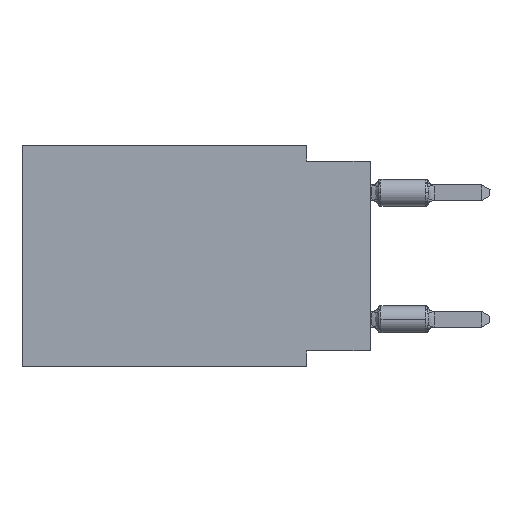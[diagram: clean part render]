
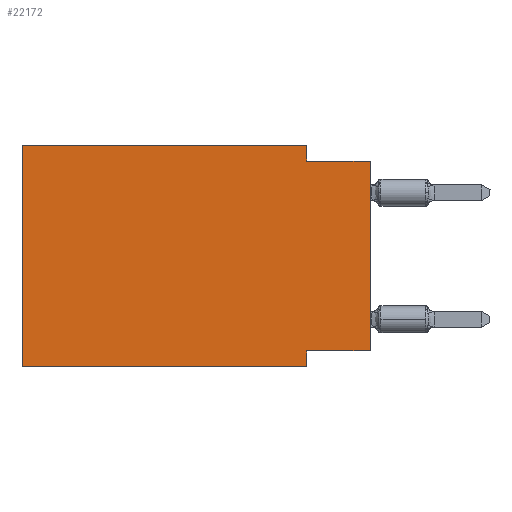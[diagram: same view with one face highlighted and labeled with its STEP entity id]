
A CAD part, left-side view. The second image highlights one B-rep face of the part: STEP entity #22172.
In plain terms, the highlighted planar face has unit normal (-1, 0, 0).
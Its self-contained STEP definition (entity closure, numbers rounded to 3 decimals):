
#338 = VECTOR ( 'NONE', #21664, 1000. ) ;
#399 = VERTEX_POINT ( 'NONE', #14264 ) ;
#623 = LINE ( 'NONE', #23967, #23879 ) ;
#987 = VERTEX_POINT ( 'NONE', #2656 ) ;
#2633 = CARTESIAN_POINT ( 'NONE',  ( 0., 13.97, 0. ) ) ;
#2656 = CARTESIAN_POINT ( 'NONE',  ( 0., 13.97, -8.89 ) ) ;
#2758 = EDGE_CURVE ( 'NONE', #3382, #399, #11212, .T. ) ;
#3339 = FACE_OUTER_BOUND ( 'NONE', #24590, .T. ) ;
#3382 = VERTEX_POINT ( 'NONE', #27331 ) ;
#3760 = VECTOR ( 'NONE', #12024, 1000. ) ;
#4665 = CARTESIAN_POINT ( 'NONE',  ( 0., 0., 0. ) ) ;
#5239 = LINE ( 'NONE', #24772, #11299 ) ;
#5345 = VERTEX_POINT ( 'NONE', #9623 ) ;
#5519 = DIRECTION ( 'NONE',  ( 0., 0., 1. ) ) ;
#6769 = VECTOR ( 'NONE', #18265, 1000. ) ;
#6833 = ORIENTED_EDGE ( 'NONE', *, *, #20634, .F. ) ;
#6986 = DIRECTION ( 'NONE',  ( 0., -1., 0. ) ) ;
#7038 = LINE ( 'NONE', #4665, #338 ) ;
#7321 = CARTESIAN_POINT ( 'NONE',  ( 0., 2.54, 0. ) ) ;
#7793 = ORIENTED_EDGE ( 'NONE', *, *, #2758, .F. ) ;
#8120 = DIRECTION ( 'NONE',  ( 0., 0., -1. ) ) ;
#8438 = ORIENTED_EDGE ( 'NONE', *, *, #23819, .F. ) ;
#8537 = EDGE_CURVE ( 'NONE', #23138, #5345, #18542, .T. ) ;
#9420 = ORIENTED_EDGE ( 'NONE', *, *, #10108, .F. ) ;
#9623 = CARTESIAN_POINT ( 'NONE',  ( 0., 2.54, -8.255 ) ) ;
#9711 = AXIS2_PLACEMENT_3D ( 'NONE', #18797, #27377, #8120 ) ;
#9841 = ORIENTED_EDGE ( 'NONE', *, *, #23227, .T. ) ;
#9898 = VECTOR ( 'NONE', #18195, 1000. ) ;
#10108 = EDGE_CURVE ( 'NONE', #399, #18042, #10135, .T. ) ;
#10135 = LINE ( 'NONE', #7321, #17429 ) ;
#11049 = DIRECTION ( 'NONE',  ( 0., -1., 0. ) ) ;
#11212 = LINE ( 'NONE', #2633, #22185 ) ;
#11299 = VECTOR ( 'NONE', #5519, 1000. ) ;
#11403 = ORIENTED_EDGE ( 'NONE', *, *, #8537, .F. ) ;
#12024 = DIRECTION ( 'NONE',  ( 0., 0., -1. ) ) ;
#12200 = CARTESIAN_POINT ( 'NONE',  ( 0., 0., -0.635 ) ) ;
#12247 = CARTESIAN_POINT ( 'NONE',  ( 0., 2.54, -8.89 ) ) ;
#14264 = CARTESIAN_POINT ( 'NONE',  ( 0., 2.54, 0. ) ) ;
#14389 = LINE ( 'NONE', #20724, #9898 ) ;
#16452 = VERTEX_POINT ( 'NONE', #12247 ) ;
#17429 = VECTOR ( 'NONE', #22637, 1000. ) ;
#17592 = ORIENTED_EDGE ( 'NONE', *, *, #17677, .F. ) ;
#17677 = EDGE_CURVE ( 'NONE', #18042, #27198, #623, .T. ) ;
#18042 = VERTEX_POINT ( 'NONE', #24445 ) ;
#18195 = DIRECTION ( 'NONE',  ( 0., -1., 0. ) ) ;
#18265 = DIRECTION ( 'NONE',  ( 0., 1., 0. ) ) ;
#18542 = LINE ( 'NONE', #26701, #6769 ) ;
#18797 = CARTESIAN_POINT ( 'NONE',  ( 0., 13.97, 0. ) ) ;
#18990 = EDGE_CURVE ( 'NONE', #987, #16452, #14389, .T. ) ;
#19153 = CARTESIAN_POINT ( 'NONE',  ( 0., 0., -8.255 ) ) ;
#19332 = ORIENTED_EDGE ( 'NONE', *, *, #18990, .T. ) ;
#20634 = EDGE_CURVE ( 'NONE', #987, #3382, #5239, .T. ) ;
#20724 = CARTESIAN_POINT ( 'NONE',  ( 0., 13.97, -8.89 ) ) ;
#21019 = CARTESIAN_POINT ( 'NONE',  ( 0., 2.54, -8.89 ) ) ;
#21664 = DIRECTION ( 'NONE',  ( 0., 0., 1. ) ) ;
#22172 = ADVANCED_FACE ( 'NONE', ( #3339 ), #24980, .F. ) ;
#22185 = VECTOR ( 'NONE', #6986, 1000. ) ;
#22637 = DIRECTION ( 'NONE',  ( 0., 0., -1. ) ) ;
#23138 = VERTEX_POINT ( 'NONE', #19153 ) ;
#23227 = EDGE_CURVE ( 'NONE', #23138, #27198, #7038, .T. ) ;
#23819 = EDGE_CURVE ( 'NONE', #5345, #16452, #25094, .T. ) ;
#23879 = VECTOR ( 'NONE', #11049, 1000. ) ;
#23967 = CARTESIAN_POINT ( 'NONE',  ( 0., 0., -0.635 ) ) ;
#24445 = CARTESIAN_POINT ( 'NONE',  ( 0., 2.54, -0.635 ) ) ;
#24590 = EDGE_LOOP ( 'NONE', ( #9841, #17592, #9420, #7793, #6833, #19332, #8438, #11403 ) ) ;
#24772 = CARTESIAN_POINT ( 'NONE',  ( 0., 13.97, 0. ) ) ;
#24980 = PLANE ( 'NONE',  #9711 ) ;
#25094 = LINE ( 'NONE', #21019, #3760 ) ;
#26701 = CARTESIAN_POINT ( 'NONE',  ( 0., 0., -8.255 ) ) ;
#27198 = VERTEX_POINT ( 'NONE', #12200 ) ;
#27331 = CARTESIAN_POINT ( 'NONE',  ( 0., 13.97, 0. ) ) ;
#27377 = DIRECTION ( 'NONE',  ( 1., 0., 0. ) ) ;
